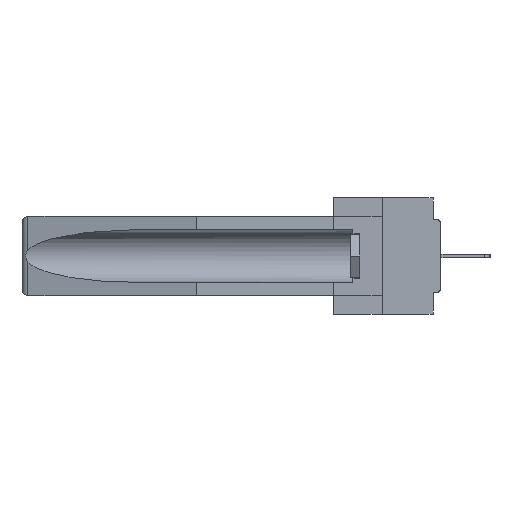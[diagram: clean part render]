
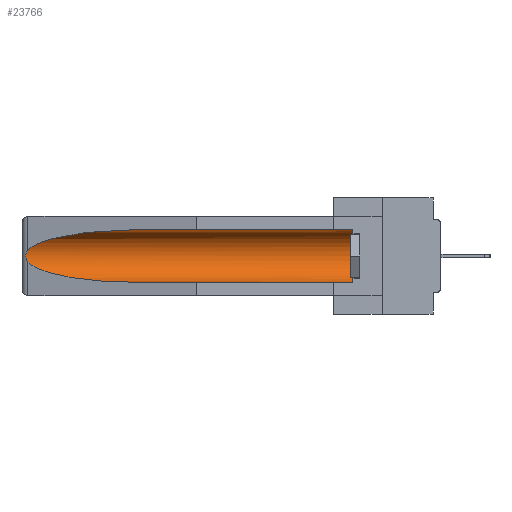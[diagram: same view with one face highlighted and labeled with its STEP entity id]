
A CAD part, left-side view. The second image highlights one B-rep face of the part: STEP entity #23766.
In plain terms, the highlighted cylindrical face has radius 2.857 mm (diameter 5.715 mm), a partial arc.
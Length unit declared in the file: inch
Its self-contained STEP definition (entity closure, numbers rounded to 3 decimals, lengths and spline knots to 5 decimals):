
#94 = CARTESIAN_POINT ( 'NONE',  ( 0.26654, 1.53092, -0.15636 ) ) ;
#630 = CARTESIAN_POINT ( 'NONE',  ( 0.155, 0.126, -0.1715 ) ) ;
#1310 = ORIENTED_EDGE ( 'NONE', *, *, #11487, .T. ) ;
#1991 = DIRECTION ( 'NONE',  ( 0., 1., 0. ) ) ;
#2357 = AXIS2_PLACEMENT_3D ( 'NONE', #29728, #1991, #39016 ) ;
#2746 = CARTESIAN_POINT ( 'NONE',  ( 0.21114, 1.30732, -0.284 ) ) ;
#2838 = VERTEX_POINT ( 'NONE', #18506 ) ;
#2863 =( BOUNDED_CURVE ( )  B_SPLINE_CURVE ( 3, ( #32925, #5199, #11114, #4793 ),
 .UNSPECIFIED., .F., .F. ) 
 B_SPLINE_CURVE_WITH_KNOTS ( ( 4, 4 ),
 ( 4.71239, 6.08839 ),
 .UNSPECIFIED. ) 
 CURVE ( )  GEOMETRIC_REPRESENTATION_ITEM ( )  RATIONAL_B_SPLINE_CURVE ( ( 1., 0.848, 0.848, 1. ) ) 
 REPRESENTATION_ITEM ( '' )  );
#3290 = CARTESIAN_POINT ( 'NONE',  ( 0.2675, 1.53308, -0.17534 ) ) ;
#4074 = ORIENTED_EDGE ( 'NONE', *, *, #18990, .T. ) ;
#4793 = CARTESIAN_POINT ( 'NONE',  ( 0.26537, 1.52718, -0.14972 ) ) ;
#5199 = CARTESIAN_POINT ( 'NONE',  ( 0.21114, 1.30732, -0.059 ) ) ;
#6496 = EDGE_CURVE ( 'NONE', #2838, #12301, #29847, .T. ) ;
#6498 = ORIENTED_EDGE ( 'NONE', *, *, #30744, .T. ) ;
#8533 = ORIENTED_EDGE ( 'NONE', *, *, #14609, .F. ) ;
#8656 = CARTESIAN_POINT ( 'NONE',  ( 0.155, 1.07973, -0.284 ) ) ;
#9424 = CARTESIAN_POINT ( 'NONE',  ( 0.26537, 1.52718, -0.14972 ) ) ;
#10182 = LINE ( 'NONE', #10973, #15892 ) ;
#10973 = CARTESIAN_POINT ( 'NONE',  ( 0.155, -0.30754, -0.284 ) ) ;
#11114 = CARTESIAN_POINT ( 'NONE',  ( 0.25451, 1.48313, -0.09465 ) ) ;
#11487 = EDGE_CURVE ( 'NONE', #31202, #30876, #24538, .T. ) ;
#12301 = VERTEX_POINT ( 'NONE', #23483 ) ;
#12596 = DIRECTION ( 'NONE',  ( 0., 0., 1. ) ) ;
#12664 = CARTESIAN_POINT ( 'NONE',  ( 0.26537, 1.52718, -0.19328 ) ) ;
#12729 =( BOUNDED_CURVE ( )  B_SPLINE_CURVE ( 3, ( #22313, #17589, #2746, #8656 ),
 .UNSPECIFIED., .F., .F. ) 
 B_SPLINE_CURVE_WITH_KNOTS ( ( 4, 4 ),
 ( 0.1948, 1.5708 ),
 .UNSPECIFIED. ) 
 CURVE ( )  GEOMETRIC_REPRESENTATION_ITEM ( )  RATIONAL_B_SPLINE_CURVE ( ( 1., 0.848, 0.848, 1. ) ) 
 REPRESENTATION_ITEM ( '' )  );
#13628 = DIRECTION ( 'NONE',  ( 0., 1., 0. ) ) ;
#14008 = EDGE_CURVE ( 'NONE', #12301, #31202, #2863, .T. ) ;
#14310 = CARTESIAN_POINT ( 'NONE',  ( 0.26537, 1.52718, -0.14972 ) ) ;
#14388 = CIRCLE ( 'NONE', #21524, 0.1125 ) ;
#14512 = DIRECTION ( 'NONE',  ( 0., 1., 0. ) ) ;
#14609 = EDGE_CURVE ( 'NONE', #24223, #29104, #10182, .T. ) ;
#15696 = CARTESIAN_POINT ( 'NONE',  ( 0.2673, 1.53269, -0.17917 ) ) ;
#15892 = VECTOR ( 'NONE', #13628, 39.37008 ) ;
#17589 = CARTESIAN_POINT ( 'NONE',  ( 0.25451, 1.48313, -0.24835 ) ) ;
#17591 = CARTESIAN_POINT ( 'NONE',  ( 0.155, 0.126, -0.284 ) ) ;
#18506 = CARTESIAN_POINT ( 'NONE',  ( 0.155, 0.126, -0.059 ) ) ;
#18715 = VECTOR ( 'NONE', #14512, 39.37008 ) ;
#18936 = CARTESIAN_POINT ( 'NONE',  ( 0.2675, 1.53308, -0.16763 ) ) ;
#18990 = EDGE_CURVE ( 'NONE', #30876, #29104, #12729, .T. ) ;
#20023 = EDGE_LOOP ( 'NONE', ( #27402, #1310, #4074, #8533, #6498, #25471 ) ) ;
#20462 = FACE_OUTER_BOUND ( 'NONE', #20023, .T. ) ;
#21524 = AXIS2_PLACEMENT_3D ( 'NONE', #630, #22113, #12596 ) ;
#22113 = DIRECTION ( 'NONE',  ( 0., -1., 0. ) ) ;
#22167 = CARTESIAN_POINT ( 'NONE',  ( 0.26655, 1.53094, -0.18657 ) ) ;
#22313 = CARTESIAN_POINT ( 'NONE',  ( 0.26537, 1.52718, -0.19328 ) ) ;
#23483 = CARTESIAN_POINT ( 'NONE',  ( 0.155, 1.07973, -0.059 ) ) ;
#23766 = ADVANCED_FACE ( 'NONE', ( #20462 ), #32761, .F. ) ;
#24223 = VERTEX_POINT ( 'NONE', #17591 ) ;
#24262 = CARTESIAN_POINT ( 'NONE',  ( 0.26537, 1.52718, -0.19328 ) ) ;
#24538 = B_SPLINE_CURVE_WITH_KNOTS ( 'NONE', 3,
 ( #9424, #33872, #94, #34072, #18936, #3290, #15696, #22167, #28406, #12664 ),
 .UNSPECIFIED., .F., .F.,
 ( 4, 2, 2, 2, 4 ),
 ( 0., 0.00029, 0.00058, 0.00087, 0.00117 ),
 .UNSPECIFIED. ) ;
#25471 = ORIENTED_EDGE ( 'NONE', *, *, #6496, .T. ) ;
#27402 = ORIENTED_EDGE ( 'NONE', *, *, #14008, .T. ) ;
#28406 = CARTESIAN_POINT ( 'NONE',  ( 0.26597, 1.5296, -0.19026 ) ) ;
#29104 = VERTEX_POINT ( 'NONE', #37074 ) ;
#29728 = CARTESIAN_POINT ( 'NONE',  ( 0.155, -0.30754, -0.1715 ) ) ;
#29847 = LINE ( 'NONE', #32298, #18715 ) ;
#30744 = EDGE_CURVE ( 'NONE', #24223, #2838, #14388, .T. ) ;
#30876 = VERTEX_POINT ( 'NONE', #24262 ) ;
#31202 = VERTEX_POINT ( 'NONE', #14310 ) ;
#32298 = CARTESIAN_POINT ( 'NONE',  ( 0.155, -0.30754, -0.059 ) ) ;
#32761 = CYLINDRICAL_SURFACE ( 'NONE', #2357, 0.1125 ) ;
#32925 = CARTESIAN_POINT ( 'NONE',  ( 0.155, 1.07973, -0.059 ) ) ;
#33872 = CARTESIAN_POINT ( 'NONE',  ( 0.26597, 1.52961, -0.15275 ) ) ;
#34072 = CARTESIAN_POINT ( 'NONE',  ( 0.2673, 1.5327, -0.16383 ) ) ;
#37074 = CARTESIAN_POINT ( 'NONE',  ( 0.155, 1.07973, -0.284 ) ) ;
#39016 = DIRECTION ( 'NONE',  ( 0., 0., 1. ) ) ;
